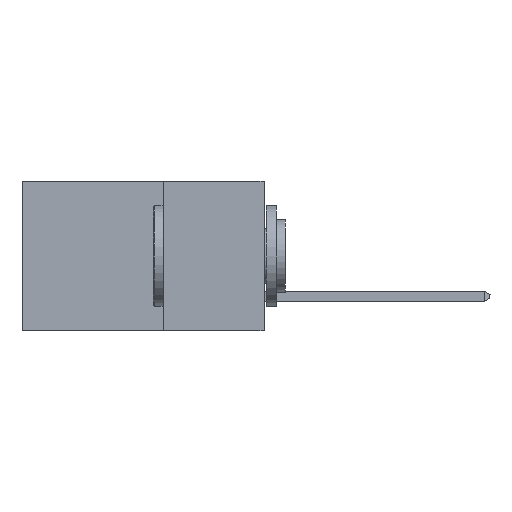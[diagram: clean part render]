
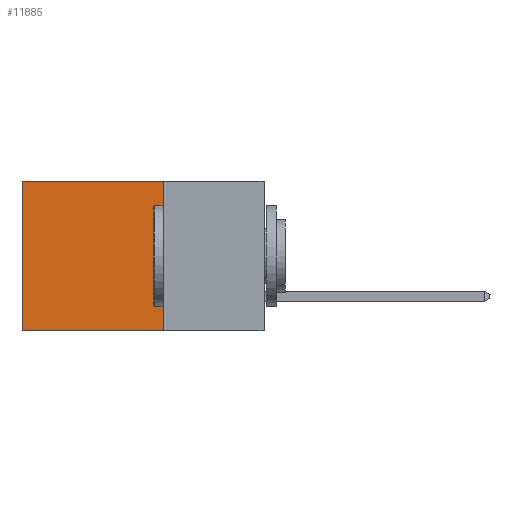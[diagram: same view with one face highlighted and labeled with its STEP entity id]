
A CAD part, left-side view. The second image highlights one B-rep face of the part: STEP entity #11885.
In plain terms, the highlighted planar face has unit normal (-1, 0, 0).
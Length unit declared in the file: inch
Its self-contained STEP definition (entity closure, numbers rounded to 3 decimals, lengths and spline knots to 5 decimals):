
#444 = DIRECTION ( 'NONE',  ( 0., 0., -1. ) ) ;
#566 = ORIENTED_EDGE ( 'NONE', *, *, #3683, .T. ) ;
#789 = LINE ( 'NONE', #3484, #5636 ) ;
#1531 = CARTESIAN_POINT ( 'NONE',  ( 0.2615, 0.6, -0.37 ) ) ;
#1794 = VECTOR ( 'NONE', #4048, 39.37008 ) ;
#2668 = DIRECTION ( 'NONE',  ( 0., 1., 0. ) ) ;
#2763 = ORIENTED_EDGE ( 'NONE', *, *, #7152, .F. ) ;
#2864 = CARTESIAN_POINT ( 'NONE',  ( 0.2615, 0.25, -0.37 ) ) ;
#3484 = CARTESIAN_POINT ( 'NONE',  ( 0.2615, 0.25, -0.37 ) ) ;
#3584 = VERTEX_POINT ( 'NONE', #1531 ) ;
#3683 = EDGE_CURVE ( 'NONE', #7034, #11152, #9950, .T. ) ;
#4048 = DIRECTION ( 'NONE',  ( 0., 0., -1. ) ) ;
#4415 = DIRECTION ( 'NONE',  ( 0., 1., 0. ) ) ;
#4593 = CARTESIAN_POINT ( 'NONE',  ( 0.2615, 0.25, -0.37 ) ) ;
#5211 = EDGE_CURVE ( 'NONE', #11152, #3584, #8743, .T. ) ;
#5367 = CARTESIAN_POINT ( 'NONE',  ( 0.2615, 0.25, 0. ) ) ;
#5636 = VECTOR ( 'NONE', #6145, 39.37008 ) ;
#5985 = LINE ( 'NONE', #4593, #6992 ) ;
#6145 = DIRECTION ( 'NONE',  ( 0., 0., -1. ) ) ;
#6161 = VERTEX_POINT ( 'NONE', #9667 ) ;
#6418 = CARTESIAN_POINT ( 'NONE',  ( 0.2615, 0.6, 0. ) ) ;
#6655 = EDGE_CURVE ( 'NONE', #6161, #3584, #5985, .T. ) ;
#6761 = CARTESIAN_POINT ( 'NONE',  ( 0.2615, 0.6, -0.37 ) ) ;
#6992 = VECTOR ( 'NONE', #4415, 39.37008 ) ;
#7034 = VERTEX_POINT ( 'NONE', #8786 ) ;
#7149 = VECTOR ( 'NONE', #2668, 39.37008 ) ;
#7152 = EDGE_CURVE ( 'NONE', #7034, #6161, #789, .T. ) ;
#7423 = FACE_OUTER_BOUND ( 'NONE', #9332, .T. ) ;
#7613 = ORIENTED_EDGE ( 'NONE', *, *, #6655, .F. ) ;
#7627 = ORIENTED_EDGE ( 'NONE', *, *, #5211, .T. ) ;
#8743 = LINE ( 'NONE', #6761, #1794 ) ;
#8786 = CARTESIAN_POINT ( 'NONE',  ( 0.2615, 0.25, 0. ) ) ;
#9332 = EDGE_LOOP ( 'NONE', ( #7627, #7613, #2763, #566 ) ) ;
#9667 = CARTESIAN_POINT ( 'NONE',  ( 0.2615, 0.25, -0.37 ) ) ;
#9715 = DIRECTION ( 'NONE',  ( 1., 0., 0. ) ) ;
#9950 = LINE ( 'NONE', #5367, #7149 ) ;
#11105 = PLANE ( 'NONE',  #11487 ) ;
#11152 = VERTEX_POINT ( 'NONE', #6418 ) ;
#11487 = AXIS2_PLACEMENT_3D ( 'NONE', #2864, #9715, #444 ) ;
#11885 = ADVANCED_FACE ( 'NONE', ( #7423 ), #11105, .F. ) ;
